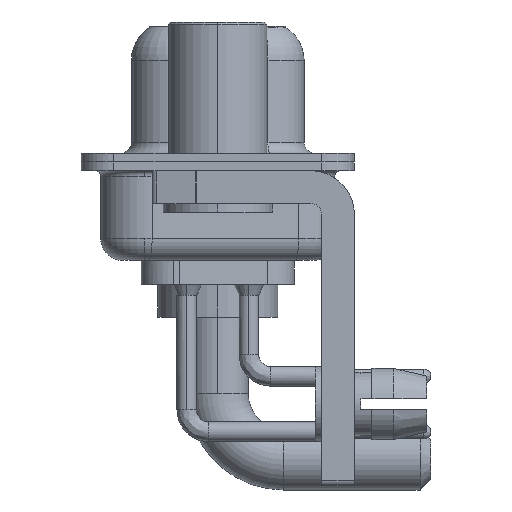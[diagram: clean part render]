
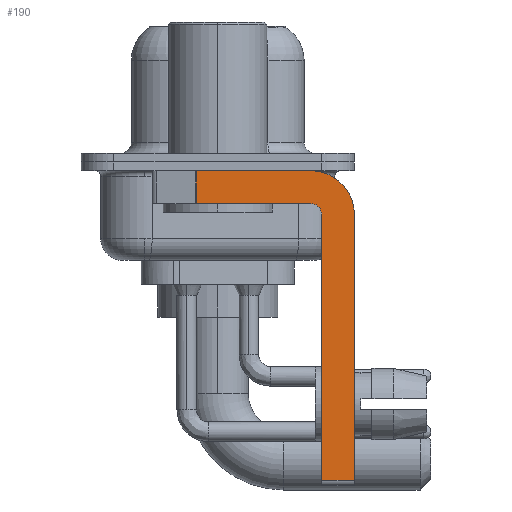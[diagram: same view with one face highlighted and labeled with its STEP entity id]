
A CAD part, left-side view. The second image highlights one B-rep face of the part: STEP entity #190.
In plain terms, the highlighted planar face has unit normal (-1, 0, 0).
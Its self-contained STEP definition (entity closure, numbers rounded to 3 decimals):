
#190 = ADVANCED_FACE ( 'NONE', ( #11388 ), #17511, .F. ) ;
#259 = LINE ( 'NONE', #4991, #15596 ) ;
#629 = LINE ( 'NONE', #14310, #19602 ) ;
#829 = DIRECTION ( 'NONE',  ( 0., 0., -1. ) ) ;
#999 = EDGE_CURVE ( 'NONE', #14994, #9574, #15235, .T. ) ;
#1274 = LINE ( 'NONE', #7418, #18619 ) ;
#1755 = ORIENTED_EDGE ( 'NONE', *, *, #17434, .F. ) ;
#2403 = CARTESIAN_POINT ( 'NONE',  ( -2.9, 0.978, -1.9 ) ) ;
#2535 = VERTEX_POINT ( 'NONE', #18933 ) ;
#3241 = VERTEX_POINT ( 'NONE', #18370 ) ;
#3473 = EDGE_LOOP ( 'NONE', ( #6178, #19341, #17066, #15257, #1755, #19682, #8230, #7901 ) ) ;
#3900 = EDGE_CURVE ( 'NONE', #3241, #14244, #259, .T. ) ;
#4927 = EDGE_CURVE ( 'NONE', #3241, #16912, #11351, .T. ) ;
#4991 = CARTESIAN_POINT ( 'NONE',  ( -2.9, 3., -0.4 ) ) ;
#5035 = VECTOR ( 'NONE', #13561, 1000. ) ;
#5042 = EDGE_CURVE ( 'NONE', #5689, #2535, #10537, .T. ) ;
#5689 = VERTEX_POINT ( 'NONE', #16931 ) ;
#6178 = ORIENTED_EDGE ( 'NONE', *, *, #3900, .F. ) ;
#6432 = CARTESIAN_POINT ( 'NONE',  ( -2.9, -6.25, -2.4 ) ) ;
#6759 = AXIS2_PLACEMENT_3D ( 'NONE', #9741, #14465, #11544 ) ;
#7072 = DIRECTION ( 'NONE',  ( 1., 0., 0. ) ) ;
#7281 = VECTOR ( 'NONE', #9849, 1000. ) ;
#7418 = CARTESIAN_POINT ( 'NONE',  ( -2.9, -4.75, -14.8 ) ) ;
#7467 = CARTESIAN_POINT ( 'NONE',  ( -2.9, -4.25, -1.9 ) ) ;
#7901 = ORIENTED_EDGE ( 'NONE', *, *, #17156, .F. ) ;
#8230 = ORIENTED_EDGE ( 'NONE', *, *, #19794, .F. ) ;
#9319 = CIRCLE ( 'NONE', #6759, 2. ) ;
#9574 = VERTEX_POINT ( 'NONE', #7467 ) ;
#9715 = DIRECTION ( 'NONE',  ( -1., 0., 0. ) ) ;
#9741 = CARTESIAN_POINT ( 'NONE',  ( -2.9, -4.25, -2.4 ) ) ;
#9849 = DIRECTION ( 'NONE',  ( 0., 0., -1. ) ) ;
#9887 = CARTESIAN_POINT ( 'NONE',  ( -2.9, -4.25, -2.4 ) ) ;
#10186 = LINE ( 'NONE', #11890, #10608 ) ;
#10537 = LINE ( 'NONE', #16661, #5035 ) ;
#10608 = VECTOR ( 'NONE', #13597, 1000. ) ;
#11351 = LINE ( 'NONE', #2403, #7281 ) ;
#11388 = FACE_OUTER_BOUND ( 'NONE', #3473, .T. ) ;
#11544 = DIRECTION ( 'NONE',  ( 0., 0., -1. ) ) ;
#11890 = CARTESIAN_POINT ( 'NONE',  ( -2.9, -4.25, -1.9 ) ) ;
#12539 = DIRECTION ( 'NONE',  ( 0., -1., 0. ) ) ;
#12836 = DIRECTION ( 'NONE',  ( 0., 0., 1. ) ) ;
#13561 = DIRECTION ( 'NONE',  ( 0., -1., 0. ) ) ;
#13597 = DIRECTION ( 'NONE',  ( 0., 1., 0. ) ) ;
#14242 = AXIS2_PLACEMENT_3D ( 'NONE', #9887, #7072, #19397 ) ;
#14244 = VERTEX_POINT ( 'NONE', #16568 ) ;
#14310 = CARTESIAN_POINT ( 'NONE',  ( -2.9, -6.25, -2.4 ) ) ;
#14465 = DIRECTION ( 'NONE',  ( 1., 0., 0. ) ) ;
#14994 = VERTEX_POINT ( 'NONE', #16016 ) ;
#15235 = CIRCLE ( 'NONE', #17777, 0.5 ) ;
#15257 = ORIENTED_EDGE ( 'NONE', *, *, #999, .F. ) ;
#15596 = VECTOR ( 'NONE', #12539, 1000. ) ;
#16016 = CARTESIAN_POINT ( 'NONE',  ( -2.9, -4.75, -2.4 ) ) ;
#16568 = CARTESIAN_POINT ( 'NONE',  ( -2.9, -4.25, -0.4 ) ) ;
#16661 = CARTESIAN_POINT ( 'NONE',  ( -2.9, -4.25, -14.55 ) ) ;
#16912 = VERTEX_POINT ( 'NONE', #17873 ) ;
#16931 = CARTESIAN_POINT ( 'NONE',  ( -2.9, -4.75, -14.55 ) ) ;
#17066 = ORIENTED_EDGE ( 'NONE', *, *, #18719, .F. ) ;
#17088 = VERTEX_POINT ( 'NONE', #6432 ) ;
#17156 = EDGE_CURVE ( 'NONE', #14244, #17088, #9319, .T. ) ;
#17340 = CARTESIAN_POINT ( 'NONE',  ( -2.9, -4.25, -2.4 ) ) ;
#17434 = EDGE_CURVE ( 'NONE', #5689, #14994, #1274, .T. ) ;
#17511 = PLANE ( 'NONE',  #14242 ) ;
#17777 = AXIS2_PLACEMENT_3D ( 'NONE', #17340, #9715, #12836 ) ;
#17873 = CARTESIAN_POINT ( 'NONE',  ( -2.9, 0.978, -1.9 ) ) ;
#18144 = DIRECTION ( 'NONE',  ( 0., 0., 1. ) ) ;
#18370 = CARTESIAN_POINT ( 'NONE',  ( -2.9, 0.978, -0.4 ) ) ;
#18619 = VECTOR ( 'NONE', #18144, 1000. ) ;
#18719 = EDGE_CURVE ( 'NONE', #9574, #16912, #10186, .T. ) ;
#18933 = CARTESIAN_POINT ( 'NONE',  ( -2.9, -6.25, -14.55 ) ) ;
#19341 = ORIENTED_EDGE ( 'NONE', *, *, #4927, .T. ) ;
#19397 = DIRECTION ( 'NONE',  ( 0., 0., -1. ) ) ;
#19602 = VECTOR ( 'NONE', #829, 1000. ) ;
#19682 = ORIENTED_EDGE ( 'NONE', *, *, #5042, .T. ) ;
#19794 = EDGE_CURVE ( 'NONE', #17088, #2535, #629, .T. ) ;
